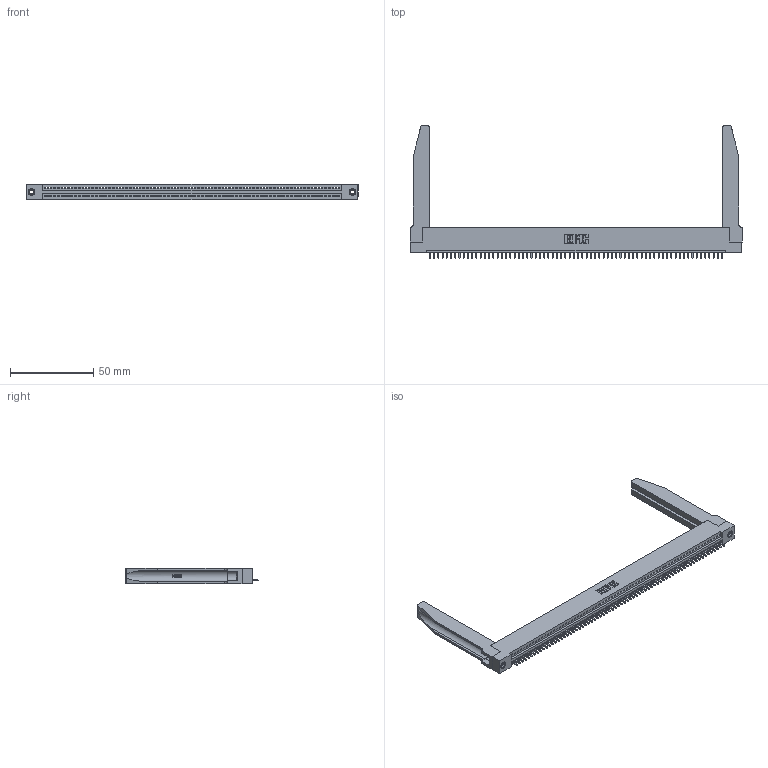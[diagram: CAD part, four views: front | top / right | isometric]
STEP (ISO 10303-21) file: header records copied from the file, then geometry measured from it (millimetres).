
FILE_DESCRIPTION (( 'STEP AP203' ), '1' );
FILE_NAME ('345-070-521-178.STEP', '2019-10-12T15:12:56', ( '' ), ( '' ), 'SwSTEP 2.0', 'SolidWorks 2016', '' );
FILE_SCHEMA (( 'CONFIG_CONTROL_DESIGN' ));
Length unit declared in the file: inch
Products named in the file (5): 345-250-001_345-250-001-102; 345 Part_Flush Mounting Lugs - 0.156 Dia-TH; 345-292-001_345-293-121; 345-220-078_345-220-078; 345-070-521-178
Assembly tree (75 placements, depth 2):
  345-070-521-178
    345 Part_Flush Mounting Lugs - 0.156 Dia-TH
    345-292-001_345-293-121  x70
    345-250-001_345-250-001-102  x2
    345-220-078_345-220-078  x2
Bounding box: 199.03 x 79.68 x 9.4 mm (x, y, z)
Volume: 26705.2 mm3; surface area: 31609.7 mm2
Topology: 75 solids, 75 shells, 4420 faces, 13269 edges, 8742 vertices
Faces by surface type: plane 3022, cylinder 1346, bspline 36, cone 12, torus 4
Entity records: 53672 total; most frequent: CARTESIAN_POINT 10193, ORIENTED_EDGE 9094, DIRECTION 7869, EDGE_CURVE 4547, LINE 4041, VECTOR 4041, VERTEX_POINT 3024, AXIS2_PLACEMENT_3D 1914
